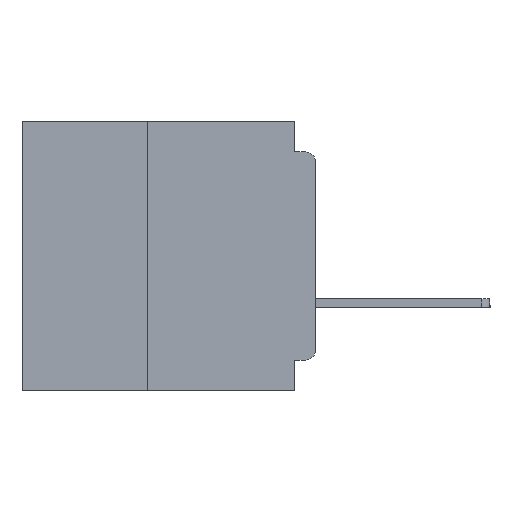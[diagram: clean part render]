
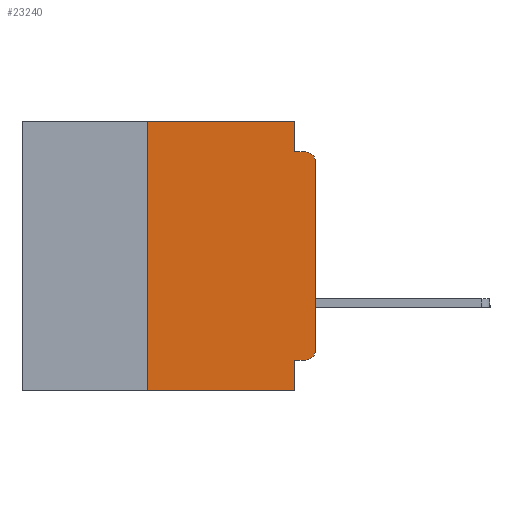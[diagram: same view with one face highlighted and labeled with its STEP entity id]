
A CAD part, left-side view. The second image highlights one B-rep face of the part: STEP entity #23240.
In plain terms, the highlighted planar face has unit normal (-1, 0, 0).
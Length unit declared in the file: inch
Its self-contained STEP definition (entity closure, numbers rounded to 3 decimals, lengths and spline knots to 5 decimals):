
#622 = CARTESIAN_POINT ( 'NONE',  ( 0., 0.437, 0. ) ) ;
#919 = CARTESIAN_POINT ( 'NONE',  ( 0., 0.015, -0.34 ) ) ;
#1316 = VERTEX_POINT ( 'NONE', #27646 ) ;
#2190 = CARTESIAN_POINT ( 'NONE',  ( 0., 0., -0.355 ) ) ;
#2431 = VERTEX_POINT ( 'NONE', #23990 ) ;
#2711 = AXIS2_PLACEMENT_3D ( 'NONE', #622, #11706, #30657 ) ;
#3023 = VERTEX_POINT ( 'NONE', #19365 ) ;
#3343 = FACE_OUTER_BOUND ( 'NONE', #10998, .T. ) ;
#3439 = PLANE ( 'NONE',  #2711 ) ;
#3496 = ORIENTED_EDGE ( 'NONE', *, *, #13609, .F. ) ;
#3724 = DIRECTION ( 'NONE',  ( 0., 0., -1. ) ) ;
#4153 = EDGE_CURVE ( 'NONE', #25508, #32782, #12602, .T. ) ;
#5677 = VECTOR ( 'NONE', #24072, 39.37008 ) ;
#5777 = VECTOR ( 'NONE', #12095, 39.37008 ) ;
#6063 = ORIENTED_EDGE ( 'NONE', *, *, #14077, .F. ) ;
#6624 = DIRECTION ( 'NONE',  ( 0., 0., 1. ) ) ;
#7755 = CARTESIAN_POINT ( 'NONE',  ( 0., 0.031, -0.355 ) ) ;
#8012 = EDGE_CURVE ( 'NONE', #2431, #24249, #14835, .T. ) ;
#8233 = VERTEX_POINT ( 'NONE', #7755 ) ;
#8933 = LINE ( 'NONE', #10257, #23444 ) ;
#9253 = LINE ( 'NONE', #30138, #16569 ) ;
#9906 = VERTEX_POINT ( 'NONE', #24044 ) ;
#10257 = CARTESIAN_POINT ( 'NONE',  ( 0., 0.031, 0. ) ) ;
#10765 = ORIENTED_EDGE ( 'NONE', *, *, #34568, .F. ) ;
#10998 = EDGE_LOOP ( 'NONE', ( #32684, #27265, #18812, #15025, #10765, #19701, #25657, #3496, #6063, #21902 ) ) ;
#11706 = DIRECTION ( 'NONE',  ( 1., 0., 0. ) ) ;
#11797 = EDGE_CURVE ( 'NONE', #2431, #9906, #31910, .T. ) ;
#12095 = DIRECTION ( 'NONE',  ( 0., -1., 0. ) ) ;
#12292 = CARTESIAN_POINT ( 'NONE',  ( 0., 0., 0. ) ) ;
#12602 = LINE ( 'NONE', #33813, #18990 ) ;
#13231 = CARTESIAN_POINT ( 'NONE',  ( 0., 0.015, -0.355 ) ) ;
#13609 = EDGE_CURVE ( 'NONE', #8233, #24249, #27815, .T. ) ;
#13682 = DIRECTION ( 'NONE',  ( 0., 0., -1. ) ) ;
#14077 = EDGE_CURVE ( 'NONE', #19391, #8233, #20219, .T. ) ;
#14118 = CARTESIAN_POINT ( 'NONE',  ( 0., 0.015, -0.06 ) ) ;
#14835 = LINE ( 'NONE', #33852, #5777 ) ;
#15025 = ORIENTED_EDGE ( 'NONE', *, *, #16129, .F. ) ;
#16129 = EDGE_CURVE ( 'NONE', #3023, #25508, #8933, .T. ) ;
#16426 = CARTESIAN_POINT ( 'NONE',  ( 0., 0.031, -0.4 ) ) ;
#16569 = VECTOR ( 'NONE', #19291, 39.37008 ) ;
#16840 = DIRECTION ( 'NONE',  ( 0., 0., -1. ) ) ;
#18458 = AXIS2_PLACEMENT_3D ( 'NONE', #14118, #32996, #16840 ) ;
#18812 = ORIENTED_EDGE ( 'NONE', *, *, #4153, .F. ) ;
#18963 = EDGE_CURVE ( 'NONE', #1316, #32782, #27502, .T. ) ;
#18990 = VECTOR ( 'NONE', #33579, 39.37008 ) ;
#19020 = CARTESIAN_POINT ( 'NONE',  ( 0., 0.25, -0.4 ) ) ;
#19156 = CARTESIAN_POINT ( 'NONE',  ( 0., 0.031, -0.4 ) ) ;
#19291 = DIRECTION ( 'NONE',  ( 0., -1., 0. ) ) ;
#19365 = CARTESIAN_POINT ( 'NONE',  ( 0., 0.031, 0. ) ) ;
#19391 = VERTEX_POINT ( 'NONE', #13231 ) ;
#19516 = VERTEX_POINT ( 'NONE', #29913 ) ;
#19643 = LINE ( 'NONE', #12292, #33124 ) ;
#19701 = ORIENTED_EDGE ( 'NONE', *, *, #11797, .F. ) ;
#20109 = DIRECTION ( 'NONE',  ( -1., 0., 0. ) ) ;
#20219 = LINE ( 'NONE', #2190, #5677 ) ;
#21726 = DIRECTION ( 'NONE',  ( 0., 0., 1. ) ) ;
#21902 = ORIENTED_EDGE ( 'NONE', *, *, #28382, .T. ) ;
#21917 = CARTESIAN_POINT ( 'NONE',  ( 0., 0.031, -0.045 ) ) ;
#22296 = AXIS2_PLACEMENT_3D ( 'NONE', #919, #20109, #3724 ) ;
#22747 = EDGE_CURVE ( 'NONE', #19516, #1316, #19643, .T. ) ;
#23240 = ADVANCED_FACE ( 'NONE', ( #3343 ), #3439, .F. ) ;
#23444 = VECTOR ( 'NONE', #29240, 39.37008 ) ;
#23990 = CARTESIAN_POINT ( 'NONE',  ( 0., 0.25, -0.4 ) ) ;
#24044 = CARTESIAN_POINT ( 'NONE',  ( 0., 0.25, 0. ) ) ;
#24072 = DIRECTION ( 'NONE',  ( 0., 1., 0. ) ) ;
#24249 = VERTEX_POINT ( 'NONE', #19156 ) ;
#24757 = VECTOR ( 'NONE', #21726, 39.37008 ) ;
#25508 = VERTEX_POINT ( 'NONE', #21917 ) ;
#25657 = ORIENTED_EDGE ( 'NONE', *, *, #8012, .T. ) ;
#27265 = ORIENTED_EDGE ( 'NONE', *, *, #18963, .T. ) ;
#27502 = CIRCLE ( 'NONE', #18458, 0.015 ) ;
#27646 = CARTESIAN_POINT ( 'NONE',  ( 0., 0., -0.06 ) ) ;
#27815 = LINE ( 'NONE', #16426, #34562 ) ;
#28382 = EDGE_CURVE ( 'NONE', #19391, #19516, #35091, .T. ) ;
#29240 = DIRECTION ( 'NONE',  ( 0., 0., -1. ) ) ;
#29913 = CARTESIAN_POINT ( 'NONE',  ( 0., 0., -0.34 ) ) ;
#30138 = CARTESIAN_POINT ( 'NONE',  ( 0., 0.437, 0. ) ) ;
#30657 = DIRECTION ( 'NONE',  ( 0., 0., -1. ) ) ;
#31910 = LINE ( 'NONE', #19020, #24757 ) ;
#32684 = ORIENTED_EDGE ( 'NONE', *, *, #22747, .T. ) ;
#32782 = VERTEX_POINT ( 'NONE', #33261 ) ;
#32996 = DIRECTION ( 'NONE',  ( -1., 0., 0. ) ) ;
#33124 = VECTOR ( 'NONE', #6624, 39.37008 ) ;
#33261 = CARTESIAN_POINT ( 'NONE',  ( 0., 0.015, -0.045 ) ) ;
#33579 = DIRECTION ( 'NONE',  ( 0., -1., 0. ) ) ;
#33813 = CARTESIAN_POINT ( 'NONE',  ( 0., 0., -0.045 ) ) ;
#33852 = CARTESIAN_POINT ( 'NONE',  ( 0., 0.437, -0.4 ) ) ;
#34562 = VECTOR ( 'NONE', #13682, 39.37008 ) ;
#34568 = EDGE_CURVE ( 'NONE', #9906, #3023, #9253, .T. ) ;
#35091 = CIRCLE ( 'NONE', #22296, 0.015 ) ;
